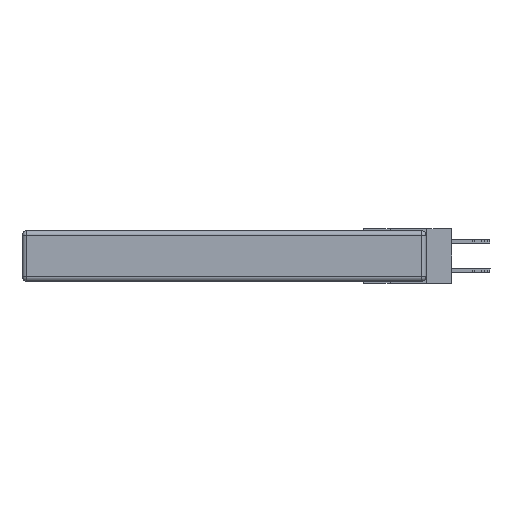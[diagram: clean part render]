
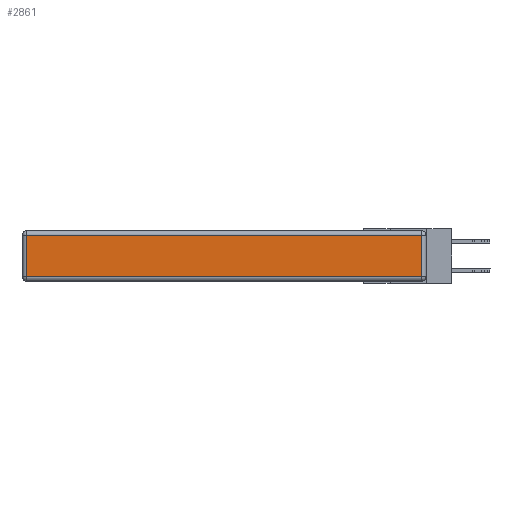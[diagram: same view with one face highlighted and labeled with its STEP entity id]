
A CAD part, left-side view. The second image highlights one B-rep face of the part: STEP entity #2861.
In plain terms, the highlighted planar face has unit normal (-1, 0, 0).
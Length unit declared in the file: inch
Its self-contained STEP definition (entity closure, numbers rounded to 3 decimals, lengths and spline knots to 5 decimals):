
#2728 = LINE ( 'NONE', #14522, #27967 ) ;
#2861 = ADVANCED_FACE ( 'NONE', ( #18635 ), #31345, .T. ) ;
#4664 = ORIENTED_EDGE ( 'NONE', *, *, #23980, .T. ) ;
#5413 = LINE ( 'NONE', #13133, #15264 ) ;
#6221 = VECTOR ( 'NONE', #25419, 39.37008 ) ;
#9849 = ORIENTED_EDGE ( 'NONE', *, *, #22663, .T. ) ;
#10260 = ORIENTED_EDGE ( 'NONE', *, *, #15169, .T. ) ;
#10937 = LINE ( 'NONE', #22676, #6221 ) ;
#12236 = ORIENTED_EDGE ( 'NONE', *, *, #32985, .T. ) ;
#13133 = CARTESIAN_POINT ( 'NONE',  ( 0., 0., -0.313 ) ) ;
#14522 = CARTESIAN_POINT ( 'NONE',  ( 0., 0.03, -0.343 ) ) ;
#15169 = EDGE_CURVE ( 'NONE', #25687, #17613, #17361, .T. ) ;
#15264 = VECTOR ( 'NONE', #29723, 39.37008 ) ;
#16656 = DIRECTION ( 'NONE',  ( -1., 0., 0. ) ) ;
#17361 = LINE ( 'NONE', #27814, #34865 ) ;
#17613 = VERTEX_POINT ( 'NONE', #28831 ) ;
#18635 = FACE_OUTER_BOUND ( 'NONE', #31271, .T. ) ;
#22663 = EDGE_CURVE ( 'NONE', #17613, #31009, #5413, .T. ) ;
#22676 = CARTESIAN_POINT ( 'NONE',  ( 0., 2.75, -0.03 ) ) ;
#23980 = EDGE_CURVE ( 'NONE', #31009, #27335, #2728, .T. ) ;
#25419 = DIRECTION ( 'NONE',  ( 0., 1., 0. ) ) ;
#25687 = VERTEX_POINT ( 'NONE', #33525 ) ;
#27148 = CARTESIAN_POINT ( 'NONE',  ( 0., 0., -0.343 ) ) ;
#27335 = VERTEX_POINT ( 'NONE', #31804 ) ;
#27626 = DIRECTION ( 'NONE',  ( 0., 0., 1. ) ) ;
#27814 = CARTESIAN_POINT ( 'NONE',  ( 0., 2.72, -0.343 ) ) ;
#27967 = VECTOR ( 'NONE', #33639, 39.37008 ) ;
#28483 = AXIS2_PLACEMENT_3D ( 'NONE', #27148, #16656, #27626 ) ;
#28831 = CARTESIAN_POINT ( 'NONE',  ( 0., 2.72, -0.313 ) ) ;
#29723 = DIRECTION ( 'NONE',  ( 0., -1., 0. ) ) ;
#30093 = DIRECTION ( 'NONE',  ( 0., 0., -1. ) ) ;
#31009 = VERTEX_POINT ( 'NONE', #32031 ) ;
#31271 = EDGE_LOOP ( 'NONE', ( #9849, #4664, #12236, #10260 ) ) ;
#31345 = PLANE ( 'NONE',  #28483 ) ;
#31804 = CARTESIAN_POINT ( 'NONE',  ( 0., 0.03, -0.03 ) ) ;
#32031 = CARTESIAN_POINT ( 'NONE',  ( 0., 0.03, -0.313 ) ) ;
#32985 = EDGE_CURVE ( 'NONE', #27335, #25687, #10937, .T. ) ;
#33525 = CARTESIAN_POINT ( 'NONE',  ( 0., 2.72, -0.03 ) ) ;
#33639 = DIRECTION ( 'NONE',  ( 0., 0., 1. ) ) ;
#34865 = VECTOR ( 'NONE', #30093, 39.37008 ) ;
